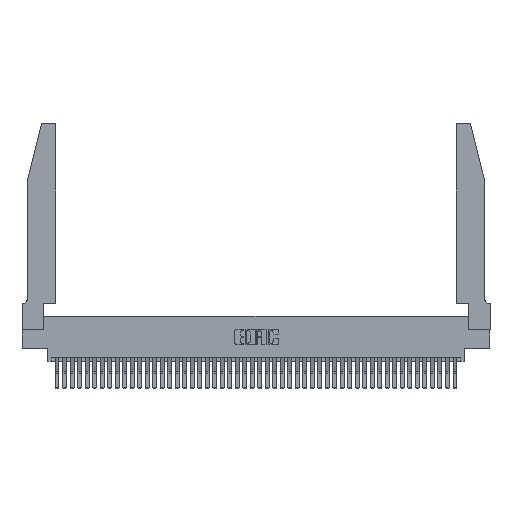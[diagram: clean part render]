
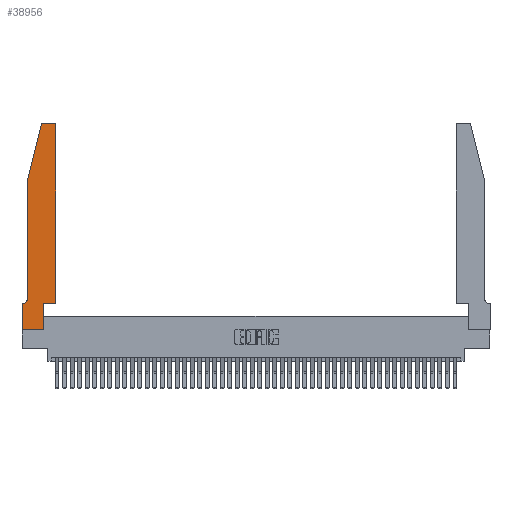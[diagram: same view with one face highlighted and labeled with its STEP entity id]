
A CAD part, top view. The second image highlights one B-rep face of the part: STEP entity #38956.
In plain terms, the highlighted planar face has unit normal (0, 0, 1).
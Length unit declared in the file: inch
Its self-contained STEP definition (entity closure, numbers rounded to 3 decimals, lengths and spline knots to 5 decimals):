
#919 = CARTESIAN_POINT ( 'NONE',  ( 0.2865, 0., 0.37 ) ) ;
#1873 = CARTESIAN_POINT ( 'NONE',  ( 0.4205, 2.75, 0.37 ) ) ;
#2254 = CARTESIAN_POINT ( 'NONE',  ( 0.284, 2.72, 0.37 ) ) ;
#2265 = ORIENTED_EDGE ( 'NONE', *, *, #30262, .T. ) ;
#2374 = CARTESIAN_POINT ( 'NONE',  ( 0.0755, 2., 0.37 ) ) ;
#2501 = VERTEX_POINT ( 'NONE', #13917 ) ;
#2705 = FACE_OUTER_BOUND ( 'NONE', #38360, .T. ) ;
#3254 = LINE ( 'NONE', #20736, #39825 ) ;
#3517 = LINE ( 'NONE', #37436, #30833 ) ;
#3974 = ORIENTED_EDGE ( 'NONE', *, *, #33706, .T. ) ;
#4982 = VECTOR ( 'NONE', #16218, 39.37008 ) ;
#5117 = VERTEX_POINT ( 'NONE', #31619 ) ;
#5341 = CARTESIAN_POINT ( 'NONE',  ( 0.0755, 2., 0.37 ) ) ;
#5458 = AXIS2_PLACEMENT_3D ( 'NONE', #21339, #45684, #24879 ) ;
#5903 = DIRECTION ( 'NONE',  ( 1., 0., 0. ) ) ;
#5979 = VERTEX_POINT ( 'NONE', #39439 ) ;
#6279 = DIRECTION ( 'NONE',  ( -1., 0., 0. ) ) ;
#7787 = EDGE_CURVE ( 'NONE', #5117, #9538, #39301, .T. ) ;
#7998 = EDGE_CURVE ( 'NONE', #43296, #43111, #3254, .T. ) ;
#8778 = LINE ( 'NONE', #25608, #26595 ) ;
#8888 = ORIENTED_EDGE ( 'NONE', *, *, #10288, .T. ) ;
#9538 = VERTEX_POINT ( 'NONE', #32081 ) ;
#9616 = VECTOR ( 'NONE', #36399, 39.37008 ) ;
#9693 = VERTEX_POINT ( 'NONE', #36628 ) ;
#10228 = ORIENTED_EDGE ( 'NONE', *, *, #35606, .T. ) ;
#10288 = EDGE_CURVE ( 'NONE', #36494, #31840, #8778, .T. ) ;
#10319 = AXIS2_PLACEMENT_3D ( 'NONE', #2254, #27261, #5903 ) ;
#10549 = PLANE ( 'NONE',  #5458 ) ;
#11225 = DIRECTION ( 'NONE',  ( 0., 0., 1. ) ) ;
#11503 = ORIENTED_EDGE ( 'NONE', *, *, #27431, .T. ) ;
#11915 = CARTESIAN_POINT ( 'NONE',  ( 0., 0.35, 0.37 ) ) ;
#12316 = CARTESIAN_POINT ( 'NONE',  ( 0.25487, 2.72718, 0.37 ) ) ;
#13594 = ORIENTED_EDGE ( 'NONE', *, *, #33890, .T. ) ;
#13908 = DIRECTION ( 'NONE',  ( 0., 1., 0. ) ) ;
#13917 = CARTESIAN_POINT ( 'NONE',  ( 0.4505, 0.35, 0.37 ) ) ;
#14572 = LINE ( 'NONE', #5341, #4982 ) ;
#14895 = DIRECTION ( 'NONE',  ( -0.239, -0.971, 0. ) ) ;
#14896 = DIRECTION ( 'NONE',  ( 0., 1., 0. ) ) ;
#16218 = DIRECTION ( 'NONE',  ( 0., -1., 0. ) ) ;
#16271 = DIRECTION ( 'NONE',  ( 1., 0., 0. ) ) ;
#16651 = VECTOR ( 'NONE', #45469, 39.37008 ) ;
#17510 = ORIENTED_EDGE ( 'NONE', *, *, #37895, .T. ) ;
#19072 = DIRECTION ( 'NONE',  ( 0., -1., 0. ) ) ;
#19663 = DIRECTION ( 'NONE',  ( 0., 0., -1. ) ) ;
#19695 = VERTEX_POINT ( 'NONE', #33463 ) ;
#20315 = ORIENTED_EDGE ( 'NONE', *, *, #34159, .T. ) ;
#20736 = CARTESIAN_POINT ( 'NONE',  ( 0.2605, 2.75, 0.37 ) ) ;
#21298 = AXIS2_PLACEMENT_3D ( 'NONE', #32405, #11225, #35916 ) ;
#21339 = CARTESIAN_POINT ( 'NONE',  ( 0., 0.35, 0.37 ) ) ;
#21375 = LINE ( 'NONE', #25888, #9616 ) ;
#21972 = CIRCLE ( 'NONE', #10319, 0.03 ) ;
#23610 = ORIENTED_EDGE ( 'NONE', *, *, #30541, .T. ) ;
#24879 = DIRECTION ( 'NONE',  ( 1., 0., 0. ) ) ;
#25484 = LINE ( 'NONE', #36525, #41820 ) ;
#25608 = CARTESIAN_POINT ( 'NONE',  ( 0.0755, 2., 0.37 ) ) ;
#25888 = CARTESIAN_POINT ( 'NONE',  ( 0., 0., 0.37 ) ) ;
#26595 = VECTOR ( 'NONE', #14895, 39.37008 ) ;
#27222 = VERTEX_POINT ( 'NONE', #11915 ) ;
#27261 = DIRECTION ( 'NONE',  ( 0., 0., 1. ) ) ;
#27431 = EDGE_CURVE ( 'NONE', #43111, #36494, #21972, .T. ) ;
#28990 = CARTESIAN_POINT ( 'NONE',  ( 0.2865, 0.35, 0.37 ) ) ;
#29611 = ORIENTED_EDGE ( 'NONE', *, *, #7787, .T. ) ;
#29807 = VECTOR ( 'NONE', #14896, 39.37008 ) ;
#30262 = EDGE_CURVE ( 'NONE', #9538, #27222, #36422, .T. ) ;
#30345 = ORIENTED_EDGE ( 'NONE', *, *, #7998, .T. ) ;
#30541 = EDGE_CURVE ( 'NONE', #27222, #5979, #25484, .T. ) ;
#30833 = VECTOR ( 'NONE', #16271, 39.37008 ) ;
#31191 = AXIS2_PLACEMENT_3D ( 'NONE', #40565, #19663, #44048 ) ;
#31511 = CARTESIAN_POINT ( 'NONE',  ( 0.4505, 0.35, 0.37 ) ) ;
#31619 = CARTESIAN_POINT ( 'NONE',  ( 0.0755, 0.42, 0.37 ) ) ;
#31750 = EDGE_CURVE ( 'NONE', #9693, #2501, #3517, .T. ) ;
#31840 = VERTEX_POINT ( 'NONE', #2374 ) ;
#32081 = CARTESIAN_POINT ( 'NONE',  ( 0.0055, 0.35, 0.37 ) ) ;
#32405 = CARTESIAN_POINT ( 'NONE',  ( 0.4205, 2.72, 0.37 ) ) ;
#33354 = LINE ( 'NONE', #31511, #41530 ) ;
#33463 = CARTESIAN_POINT ( 'NONE',  ( 0.4505, 2.72, 0.37 ) ) ;
#33706 = EDGE_CURVE ( 'NONE', #2501, #19695, #33354, .T. ) ;
#33890 = EDGE_CURVE ( 'NONE', #19695, #43296, #44212, .T. ) ;
#34159 = EDGE_CURVE ( 'NONE', #31840, #5117, #14572, .T. ) ;
#35013 = VERTEX_POINT ( 'NONE', #919 ) ;
#35606 = EDGE_CURVE ( 'NONE', #35013, #9693, #39056, .T. ) ;
#35916 = DIRECTION ( 'NONE',  ( 1., 0., 0. ) ) ;
#36399 = DIRECTION ( 'NONE',  ( 1., 0., 0. ) ) ;
#36422 = LINE ( 'NONE', #42010, #16651 ) ;
#36494 = VERTEX_POINT ( 'NONE', #12316 ) ;
#36525 = CARTESIAN_POINT ( 'NONE',  ( 0., 0., 0.37 ) ) ;
#36628 = CARTESIAN_POINT ( 'NONE',  ( 0.2865, 0.35, 0.37 ) ) ;
#37436 = CARTESIAN_POINT ( 'NONE',  ( 0.4505, 0.35, 0.37 ) ) ;
#37895 = EDGE_CURVE ( 'NONE', #5979, #35013, #21375, .T. ) ;
#38347 = ORIENTED_EDGE ( 'NONE', *, *, #31750, .T. ) ;
#38360 = EDGE_LOOP ( 'NONE', ( #30345, #11503, #8888, #20315, #29611, #2265, #23610, #17510, #10228, #38347, #3974, #13594 ) ) ;
#38956 = ADVANCED_FACE ( 'NONE', ( #2705 ), #10549, .T. ) ;
#39056 = LINE ( 'NONE', #28990, #29807 ) ;
#39301 = CIRCLE ( 'NONE', #31191, 0.07 ) ;
#39439 = CARTESIAN_POINT ( 'NONE',  ( 0., 0., 0.37 ) ) ;
#39825 = VECTOR ( 'NONE', #6279, 39.37008 ) ;
#40565 = CARTESIAN_POINT ( 'NONE',  ( 0.0055, 0.42, 0.37 ) ) ;
#41530 = VECTOR ( 'NONE', #13908, 39.37008 ) ;
#41820 = VECTOR ( 'NONE', #19072, 39.37008 ) ;
#42010 = CARTESIAN_POINT ( 'NONE',  ( 0.0755, 0.35, 0.37 ) ) ;
#43111 = VERTEX_POINT ( 'NONE', #43341 ) ;
#43296 = VERTEX_POINT ( 'NONE', #1873 ) ;
#43341 = CARTESIAN_POINT ( 'NONE',  ( 0.284, 2.75, 0.37 ) ) ;
#44048 = DIRECTION ( 'NONE',  ( -1., 0., 0. ) ) ;
#44212 = CIRCLE ( 'NONE', #21298, 0.03 ) ;
#45469 = DIRECTION ( 'NONE',  ( -1., 0., 0. ) ) ;
#45684 = DIRECTION ( 'NONE',  ( 0., 0., 1. ) ) ;
